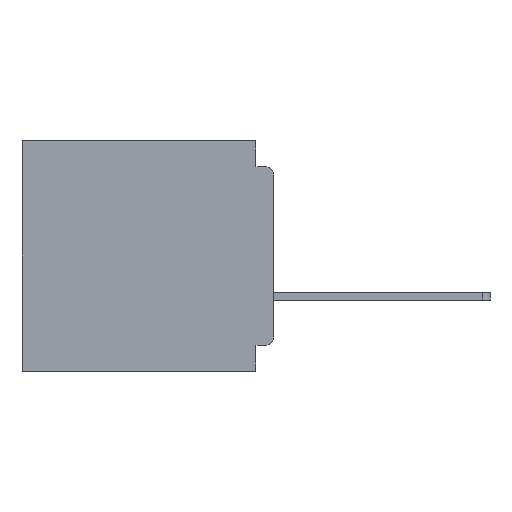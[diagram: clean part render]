
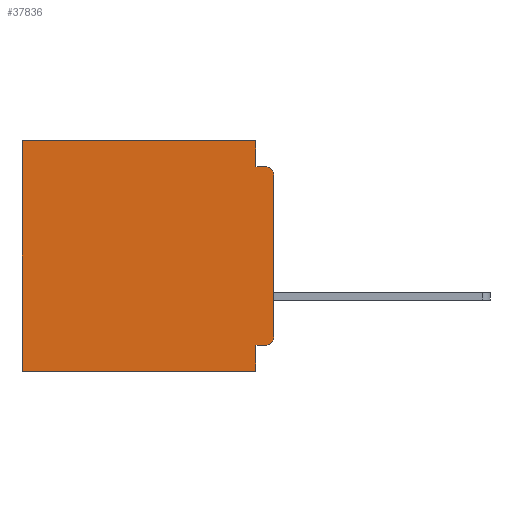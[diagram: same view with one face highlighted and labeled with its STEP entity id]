
A CAD part, left-side view. The second image highlights one B-rep face of the part: STEP entity #37836.
In plain terms, the highlighted planar face has unit normal (-1, 0, 0).
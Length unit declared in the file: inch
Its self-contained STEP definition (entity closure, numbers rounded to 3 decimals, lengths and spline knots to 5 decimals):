
#58 = VERTEX_POINT ( 'NONE', #11985 ) ;
#1053 = CARTESIAN_POINT ( 'NONE',  ( 0.3, 0.015, -0.06 ) ) ;
#2012 = CARTESIAN_POINT ( 'NONE',  ( 0.3, 0.031, -0.045 ) ) ;
#2787 = CARTESIAN_POINT ( 'NONE',  ( 0.3, 0., -0.045 ) ) ;
#3044 = VERTEX_POINT ( 'NONE', #46560 ) ;
#3169 = VECTOR ( 'NONE', #53929, 39.37008 ) ;
#3404 = CARTESIAN_POINT ( 'NONE',  ( 0.3, 0.031, -0.4 ) ) ;
#3581 = FACE_OUTER_BOUND ( 'NONE', #28590, .T. ) ;
#4072 = CARTESIAN_POINT ( 'NONE',  ( 0.3, 0., -0.355 ) ) ;
#4153 = CARTESIAN_POINT ( 'NONE',  ( 0.3, 0.015, -0.355 ) ) ;
#5271 = DIRECTION ( 'NONE',  ( 0., 0., -1. ) ) ;
#5950 = VECTOR ( 'NONE', #12151, 39.37008 ) ;
#7460 = EDGE_CURVE ( 'NONE', #17031, #49704, #16571, .T. ) ;
#7906 = CARTESIAN_POINT ( 'NONE',  ( 0.3, 0., -0.4 ) ) ;
#8044 = CARTESIAN_POINT ( 'NONE',  ( 0.3, 0.015, -0.34 ) ) ;
#8857 = EDGE_CURVE ( 'NONE', #48691, #49704, #29554, .T. ) ;
#8869 = PLANE ( 'NONE',  #45857 ) ;
#9143 = AXIS2_PLACEMENT_3D ( 'NONE', #8044, #37450, #12290 ) ;
#11709 = LINE ( 'NONE', #44391, #43877 ) ;
#11808 = VERTEX_POINT ( 'NONE', #53503 ) ;
#11985 = CARTESIAN_POINT ( 'NONE',  ( 0.3, 0.437, 0. ) ) ;
#12151 = DIRECTION ( 'NONE',  ( 0., 1., 0. ) ) ;
#12290 = DIRECTION ( 'NONE',  ( 0., 0., -1. ) ) ;
#13100 = DIRECTION ( 'NONE',  ( 1., 0., 0. ) ) ;
#16571 = CIRCLE ( 'NONE', #9143, 0.015 ) ;
#16959 = EDGE_CURVE ( 'NONE', #11808, #38114, #25570, .T. ) ;
#17031 = VERTEX_POINT ( 'NONE', #4153 ) ;
#17136 = LINE ( 'NONE', #7906, #5950 ) ;
#17268 = AXIS2_PLACEMENT_3D ( 'NONE', #1053, #30471, #5271 ) ;
#17464 = EDGE_CURVE ( 'NONE', #27951, #47341, #11709, .T. ) ;
#17573 = VECTOR ( 'NONE', #48774, 39.37008 ) ;
#18613 = VECTOR ( 'NONE', #45953, 39.37008 ) ;
#21847 = CARTESIAN_POINT ( 'NONE',  ( 0.3, 0., -0.34 ) ) ;
#22259 = ORIENTED_EDGE ( 'NONE', *, *, #44869, .F. ) ;
#22669 = CARTESIAN_POINT ( 'NONE',  ( 0.3, 0., -0.06 ) ) ;
#23014 = ORIENTED_EDGE ( 'NONE', *, *, #7460, .T. ) ;
#23499 = DIRECTION ( 'NONE',  ( 0., 0., -1. ) ) ;
#24726 = VECTOR ( 'NONE', #51836, 39.37008 ) ;
#25570 = LINE ( 'NONE', #49723, #3169 ) ;
#26494 = CARTESIAN_POINT ( 'NONE',  ( 0.3, 0., -0.4 ) ) ;
#26638 = CARTESIAN_POINT ( 'NONE',  ( 0.3, 0.015, -0.045 ) ) ;
#26681 = LINE ( 'NONE', #2787, #48966 ) ;
#27951 = VERTEX_POINT ( 'NONE', #53196 ) ;
#28507 = ORIENTED_EDGE ( 'NONE', *, *, #53140, .F. ) ;
#28590 = EDGE_LOOP ( 'NONE', ( #39016, #52387, #28757, #46923, #44034, #40286, #28507, #39889, #22259, #23014 ) ) ;
#28757 = ORIENTED_EDGE ( 'NONE', *, *, #47838, .F. ) ;
#29076 = VERTEX_POINT ( 'NONE', #26638 ) ;
#29554 = LINE ( 'NONE', #26494, #51831 ) ;
#30471 = DIRECTION ( 'NONE',  ( -1., 0., 0. ) ) ;
#30713 = DIRECTION ( 'NONE',  ( 0., 0., -1. ) ) ;
#30973 = CARTESIAN_POINT ( 'NONE',  ( 0.3, 0., 0. ) ) ;
#31089 = LINE ( 'NONE', #4072, #18613 ) ;
#32207 = DIRECTION ( 'NONE',  ( 0., -1., 0. ) ) ;
#37407 = EDGE_CURVE ( 'NONE', #11808, #58, #47016, .T. ) ;
#37450 = DIRECTION ( 'NONE',  ( -1., 0., 0. ) ) ;
#37836 = ADVANCED_FACE ( 'NONE', ( #3581 ), #8869, .F. ) ;
#38114 = VERTEX_POINT ( 'NONE', #2012 ) ;
#38259 = CARTESIAN_POINT ( 'NONE',  ( 0.3, 0., -0.4 ) ) ;
#39016 = ORIENTED_EDGE ( 'NONE', *, *, #8857, .F. ) ;
#39889 = ORIENTED_EDGE ( 'NONE', *, *, #17464, .F. ) ;
#40286 = ORIENTED_EDGE ( 'NONE', *, *, #47196, .T. ) ;
#41219 = LINE ( 'NONE', #44572, #17573 ) ;
#42454 = DIRECTION ( 'NONE',  ( 0., 0., -1. ) ) ;
#43877 = VECTOR ( 'NONE', #23499, 39.37008 ) ;
#44034 = ORIENTED_EDGE ( 'NONE', *, *, #37407, .T. ) ;
#44391 = CARTESIAN_POINT ( 'NONE',  ( 0.3, 0.031, -0.4 ) ) ;
#44572 = CARTESIAN_POINT ( 'NONE',  ( 0.3, 0.437, -0.4 ) ) ;
#44869 = EDGE_CURVE ( 'NONE', #17031, #27951, #31089, .T. ) ;
#45857 = AXIS2_PLACEMENT_3D ( 'NONE', #38259, #13100, #42454 ) ;
#45953 = DIRECTION ( 'NONE',  ( 0., 1., 0. ) ) ;
#46560 = CARTESIAN_POINT ( 'NONE',  ( 0.3, 0.437, -0.4 ) ) ;
#46923 = ORIENTED_EDGE ( 'NONE', *, *, #16959, .F. ) ;
#47016 = LINE ( 'NONE', #30973, #24726 ) ;
#47196 = EDGE_CURVE ( 'NONE', #58, #3044, #41219, .T. ) ;
#47341 = VERTEX_POINT ( 'NONE', #3404 ) ;
#47838 = EDGE_CURVE ( 'NONE', #38114, #29076, #26681, .T. ) ;
#48691 = VERTEX_POINT ( 'NONE', #22669 ) ;
#48774 = DIRECTION ( 'NONE',  ( 0., 0., -1. ) ) ;
#48966 = VECTOR ( 'NONE', #32207, 39.37008 ) ;
#49387 = CIRCLE ( 'NONE', #17268, 0.015 ) ;
#49704 = VERTEX_POINT ( 'NONE', #21847 ) ;
#49723 = CARTESIAN_POINT ( 'NONE',  ( 0.3, 0.031, 0. ) ) ;
#49738 = EDGE_CURVE ( 'NONE', #48691, #29076, #49387, .T. ) ;
#51831 = VECTOR ( 'NONE', #30713, 39.37008 ) ;
#51836 = DIRECTION ( 'NONE',  ( 0., 1., 0. ) ) ;
#52387 = ORIENTED_EDGE ( 'NONE', *, *, #49738, .T. ) ;
#53140 = EDGE_CURVE ( 'NONE', #47341, #3044, #17136, .T. ) ;
#53196 = CARTESIAN_POINT ( 'NONE',  ( 0.3, 0.031, -0.355 ) ) ;
#53503 = CARTESIAN_POINT ( 'NONE',  ( 0.3, 0.031, 0. ) ) ;
#53929 = DIRECTION ( 'NONE',  ( 0., 0., -1. ) ) ;
